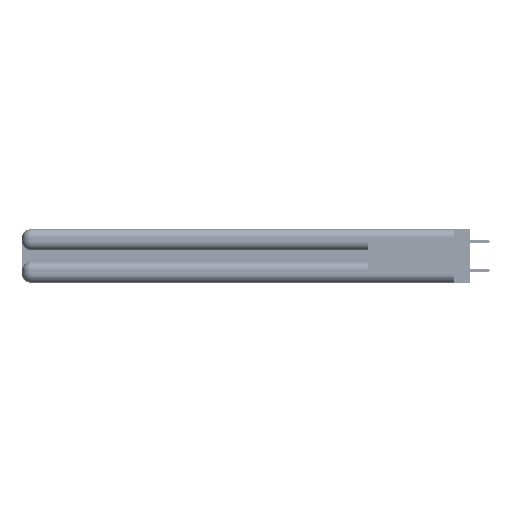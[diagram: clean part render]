
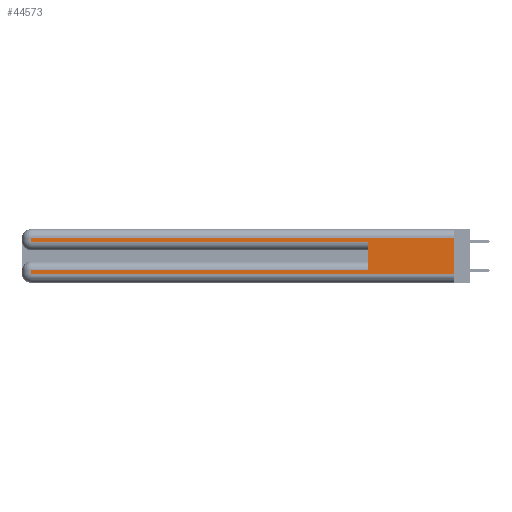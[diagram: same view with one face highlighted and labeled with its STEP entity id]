
A CAD part, left-side view. The second image highlights one B-rep face of the part: STEP entity #44573.
In plain terms, the highlighted planar face has unit normal (-1, 0, 0).
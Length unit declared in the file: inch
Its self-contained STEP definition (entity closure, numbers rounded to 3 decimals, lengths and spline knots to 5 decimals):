
#429 = AXIS2_PLACEMENT_3D ( 'NONE', #41974, #37651, #46260 ) ;
#850 = ORIENTED_EDGE ( 'NONE', *, *, #18889, .F. ) ;
#1104 = EDGE_CURVE ( 'NONE', #45478, #47218, #14773, .T. ) ;
#1220 = VECTOR ( 'NONE', #29768, 39.37008 ) ;
#1584 = CARTESIAN_POINT ( 'NONE',  ( 0., 0., 0.06 ) ) ;
#3899 = EDGE_CURVE ( 'NONE', #49265, #40483, #31799, .T. ) ;
#4111 = ORIENTED_EDGE ( 'NONE', *, *, #34907, .F. ) ;
#5415 = ORIENTED_EDGE ( 'NONE', *, *, #18656, .T. ) ;
#5717 = DIRECTION ( 'NONE',  ( 0., 0., -1. ) ) ;
#6419 = CARTESIAN_POINT ( 'NONE',  ( 0., 2.94, 0.37 ) ) ;
#8259 = LINE ( 'NONE', #12575, #1220 ) ;
#8406 = ORIENTED_EDGE ( 'NONE', *, *, #29520, .T. ) ;
#12160 = EDGE_CURVE ( 'NONE', #23995, #53709, #13234, .T. ) ;
#12575 = CARTESIAN_POINT ( 'NONE',  ( 0., 0.6, 0.145 ) ) ;
#12984 = CARTESIAN_POINT ( 'NONE',  ( 0., 2.94, 0.285 ) ) ;
#13234 = LINE ( 'NONE', #21821, #44157 ) ;
#14339 = DIRECTION ( 'NONE',  ( 0., -1., 0. ) ) ;
#14773 = LINE ( 'NONE', #19353, #21676 ) ;
#15622 = FACE_OUTER_BOUND ( 'NONE', #27334, .T. ) ;
#18656 = EDGE_CURVE ( 'NONE', #47218, #53723, #41922, .T. ) ;
#18889 = EDGE_CURVE ( 'NONE', #49265, #35035, #33871, .T. ) ;
#19198 = LINE ( 'NONE', #32373, #39328 ) ;
#19353 = CARTESIAN_POINT ( 'NONE',  ( 0., 0., 0.085 ) ) ;
#21676 = VECTOR ( 'NONE', #40539, 39.37008 ) ;
#21821 = CARTESIAN_POINT ( 'NONE',  ( 0., 0., 0.285 ) ) ;
#22454 = VECTOR ( 'NONE', #22644, 39.37008 ) ;
#22644 = DIRECTION ( 'NONE',  ( 0., 1., 0. ) ) ;
#23995 = VERTEX_POINT ( 'NONE', #12984 ) ;
#24322 = CARTESIAN_POINT ( 'NONE',  ( 0., 2.94, 0.085 ) ) ;
#24594 = CARTESIAN_POINT ( 'NONE',  ( 0., 2.94, 0.06 ) ) ;
#25375 = CARTESIAN_POINT ( 'NONE',  ( 0., 2.94, 0.31 ) ) ;
#25440 = CARTESIAN_POINT ( 'NONE',  ( 0., 0.6, 0.285 ) ) ;
#26011 = ORIENTED_EDGE ( 'NONE', *, *, #42833, .T. ) ;
#26147 = DIRECTION ( 'NONE',  ( 0., 0., -1. ) ) ;
#27334 = EDGE_LOOP ( 'NONE', ( #850, #38205, #26011, #51800, #4111, #34168, #5415, #8406 ) ) ;
#28816 = PLANE ( 'NONE',  #429 ) ;
#29520 = EDGE_CURVE ( 'NONE', #53723, #35035, #19198, .T. ) ;
#29768 = DIRECTION ( 'NONE',  ( 0., 0., 1. ) ) ;
#31799 = LINE ( 'NONE', #44949, #22454 ) ;
#32373 = CARTESIAN_POINT ( 'NONE',  ( 0., 0., 0.06 ) ) ;
#32486 = DIRECTION ( 'NONE',  ( 0., 0., -1. ) ) ;
#33871 = LINE ( 'NONE', #35573, #36312 ) ;
#34168 = ORIENTED_EDGE ( 'NONE', *, *, #1104, .T. ) ;
#34417 = DIRECTION ( 'NONE',  ( 0., -1., 0. ) ) ;
#34907 = EDGE_CURVE ( 'NONE', #45478, #53709, #8259, .T. ) ;
#35035 = VERTEX_POINT ( 'NONE', #1584 ) ;
#35516 = CARTESIAN_POINT ( 'NONE',  ( 0., 2.94, 0.37 ) ) ;
#35573 = CARTESIAN_POINT ( 'NONE',  ( 0., 0., 0.37 ) ) ;
#36063 = LINE ( 'NONE', #35516, #48763 ) ;
#36312 = VECTOR ( 'NONE', #26147, 39.37008 ) ;
#37651 = DIRECTION ( 'NONE',  ( 1., 0., 0. ) ) ;
#37738 = CARTESIAN_POINT ( 'NONE',  ( 0., 0., 0.31 ) ) ;
#38205 = ORIENTED_EDGE ( 'NONE', *, *, #3899, .T. ) ;
#39328 = VECTOR ( 'NONE', #14339, 39.37008 ) ;
#40483 = VERTEX_POINT ( 'NONE', #25375 ) ;
#40539 = DIRECTION ( 'NONE',  ( 0., 1., 0. ) ) ;
#41922 = LINE ( 'NONE', #6419, #55535 ) ;
#41974 = CARTESIAN_POINT ( 'NONE',  ( 0., 0., 0.37 ) ) ;
#42833 = EDGE_CURVE ( 'NONE', #40483, #23995, #36063, .T. ) ;
#44157 = VECTOR ( 'NONE', #34417, 39.37008 ) ;
#44573 = ADVANCED_FACE ( 'NONE', ( #15622 ), #28816, .F. ) ;
#44949 = CARTESIAN_POINT ( 'NONE',  ( 0., 0., 0.31 ) ) ;
#45478 = VERTEX_POINT ( 'NONE', #47538 ) ;
#46260 = DIRECTION ( 'NONE',  ( 0., 0., -1. ) ) ;
#47218 = VERTEX_POINT ( 'NONE', #24322 ) ;
#47538 = CARTESIAN_POINT ( 'NONE',  ( 0., 0.6, 0.085 ) ) ;
#48763 = VECTOR ( 'NONE', #5717, 39.37008 ) ;
#49265 = VERTEX_POINT ( 'NONE', #37738 ) ;
#51800 = ORIENTED_EDGE ( 'NONE', *, *, #12160, .T. ) ;
#53709 = VERTEX_POINT ( 'NONE', #25440 ) ;
#53723 = VERTEX_POINT ( 'NONE', #24594 ) ;
#55535 = VECTOR ( 'NONE', #32486, 39.37008 ) ;
